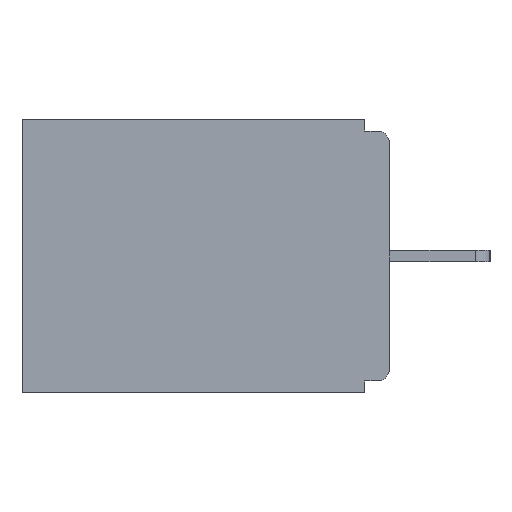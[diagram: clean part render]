
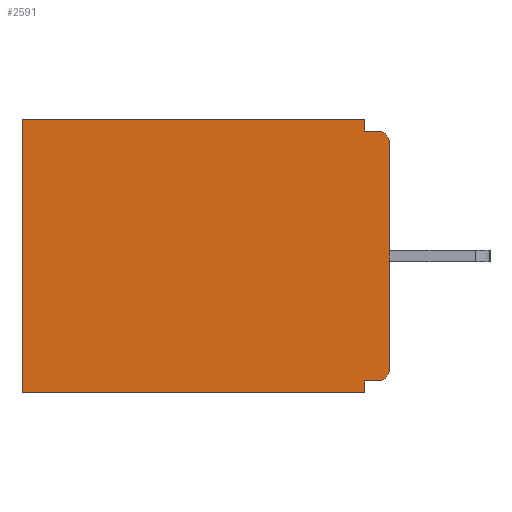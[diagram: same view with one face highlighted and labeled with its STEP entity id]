
A CAD part, left-side view. The second image highlights one B-rep face of the part: STEP entity #2591.
In plain terms, the highlighted planar face has unit normal (-1, 0, 0).
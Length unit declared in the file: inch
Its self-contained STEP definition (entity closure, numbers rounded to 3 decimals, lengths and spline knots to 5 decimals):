
#79 = CARTESIAN_POINT ( 'NONE',  ( 0.298, 0.46, 0. ) ) ;
#199 = DIRECTION ( 'NONE',  ( -1., 0., 0. ) ) ;
#314 = VERTEX_POINT ( 'NONE', #15099 ) ;
#476 = ORIENTED_EDGE ( 'NONE', *, *, #7263, .T. ) ;
#1006 = VERTEX_POINT ( 'NONE', #6099 ) ;
#1531 = EDGE_CURVE ( 'NONE', #8260, #1006, #11961, .T. ) ;
#1885 = DIRECTION ( 'NONE',  ( 0., 0., -1. ) ) ;
#2312 = CARTESIAN_POINT ( 'NONE',  ( 0.298, 0.015, -0.015 ) ) ;
#2591 = ADVANCED_FACE ( 'NONE', ( #6308 ), #11884, .F. ) ;
#3082 = EDGE_CURVE ( 'NONE', #9633, #1006, #24263, .T. ) ;
#3102 = LINE ( 'NONE', #5158, #8505 ) ;
#3244 = AXIS2_PLACEMENT_3D ( 'NONE', #20915, #3994, #19558 ) ;
#3994 = DIRECTION ( 'NONE',  ( 1., 0., 0. ) ) ;
#4077 = ORIENTED_EDGE ( 'NONE', *, *, #24033, .T. ) ;
#4218 = VERTEX_POINT ( 'NONE', #12440 ) ;
#4255 = LINE ( 'NONE', #21909, #19142 ) ;
#4772 = VECTOR ( 'NONE', #18007, 39.37008 ) ;
#4862 = EDGE_CURVE ( 'NONE', #21817, #15502, #5977, .T. ) ;
#5064 = CARTESIAN_POINT ( 'NONE',  ( 0.298, 0., -0.03 ) ) ;
#5158 = CARTESIAN_POINT ( 'NONE',  ( 0.298, 0., 0. ) ) ;
#5640 = ORIENTED_EDGE ( 'NONE', *, *, #14092, .F. ) ;
#5712 = DIRECTION ( 'NONE',  ( 0., 0., -1. ) ) ;
#5977 = LINE ( 'NONE', #21067, #17049 ) ;
#6099 = CARTESIAN_POINT ( 'NONE',  ( 0.298, 0.46, -0.343 ) ) ;
#6211 = CARTESIAN_POINT ( 'NONE',  ( 0.298, 0.031, -0.343 ) ) ;
#6308 = FACE_OUTER_BOUND ( 'NONE', #7611, .T. ) ;
#6361 = AXIS2_PLACEMENT_3D ( 'NONE', #16850, #199, #18939 ) ;
#6556 = CARTESIAN_POINT ( 'NONE',  ( 0.298, 0.031, -0.343 ) ) ;
#7172 = DIRECTION ( 'NONE',  ( -1., 0., 0. ) ) ;
#7263 = EDGE_CURVE ( 'NONE', #314, #9633, #4255, .T. ) ;
#7306 = LINE ( 'NONE', #20403, #14202 ) ;
#7573 = CIRCLE ( 'NONE', #6361, 0.015 ) ;
#7611 = EDGE_LOOP ( 'NONE', ( #19994, #12827, #5640, #476, #18282, #20814, #7846, #9367, #4077, #16255 ) ) ;
#7846 = ORIENTED_EDGE ( 'NONE', *, *, #21912, .F. ) ;
#8206 = CARTESIAN_POINT ( 'NONE',  ( 0.298, 0., -0.328 ) ) ;
#8260 = VERTEX_POINT ( 'NONE', #6211 ) ;
#8505 = VECTOR ( 'NONE', #20128, 39.37008 ) ;
#8909 = CARTESIAN_POINT ( 'NONE',  ( 0.298, 0.015, -0.03 ) ) ;
#9367 = ORIENTED_EDGE ( 'NONE', *, *, #18081, .F. ) ;
#9633 = VERTEX_POINT ( 'NONE', #18733 ) ;
#9982 = EDGE_CURVE ( 'NONE', #17358, #15502, #12496, .T. ) ;
#10052 = DIRECTION ( 'NONE',  ( 0., 1., 0. ) ) ;
#11884 = PLANE ( 'NONE',  #3244 ) ;
#11961 = LINE ( 'NONE', #17741, #4772 ) ;
#12107 = AXIS2_PLACEMENT_3D ( 'NONE', #8909, #7172, #14703 ) ;
#12270 = LINE ( 'NONE', #8206, #17140 ) ;
#12440 = CARTESIAN_POINT ( 'NONE',  ( 0.298, 0.015, -0.328 ) ) ;
#12496 = CIRCLE ( 'NONE', #12107, 0.015 ) ;
#12827 = ORIENTED_EDGE ( 'NONE', *, *, #4862, .F. ) ;
#13541 = VERTEX_POINT ( 'NONE', #20311 ) ;
#14092 = EDGE_CURVE ( 'NONE', #314, #21817, #7306, .T. ) ;
#14202 = VECTOR ( 'NONE', #1885, 39.37008 ) ;
#14595 = DIRECTION ( 'NONE',  ( 0., 1., 0. ) ) ;
#14703 = DIRECTION ( 'NONE',  ( 0., 0., -1. ) ) ;
#14843 = VECTOR ( 'NONE', #17553, 39.37008 ) ;
#15099 = CARTESIAN_POINT ( 'NONE',  ( 0.298, 0.031, 0. ) ) ;
#15502 = VERTEX_POINT ( 'NONE', #2312 ) ;
#15691 = CARTESIAN_POINT ( 'NONE',  ( 0.298, 0.031, -0.328 ) ) ;
#15722 = LINE ( 'NONE', #6556, #14843 ) ;
#16255 = ORIENTED_EDGE ( 'NONE', *, *, #19085, .F. ) ;
#16850 = CARTESIAN_POINT ( 'NONE',  ( 0.298, 0.015, -0.313 ) ) ;
#17049 = VECTOR ( 'NONE', #23396, 39.37008 ) ;
#17140 = VECTOR ( 'NONE', #10052, 39.37008 ) ;
#17358 = VERTEX_POINT ( 'NONE', #5064 ) ;
#17553 = DIRECTION ( 'NONE',  ( 0., 0., -1. ) ) ;
#17741 = CARTESIAN_POINT ( 'NONE',  ( 0.298, 0., -0.343 ) ) ;
#18007 = DIRECTION ( 'NONE',  ( 0., 1., 0. ) ) ;
#18081 = EDGE_CURVE ( 'NONE', #4218, #22318, #12270, .T. ) ;
#18228 = VECTOR ( 'NONE', #5712, 39.37008 ) ;
#18282 = ORIENTED_EDGE ( 'NONE', *, *, #3082, .T. ) ;
#18733 = CARTESIAN_POINT ( 'NONE',  ( 0.298, 0.46, 0. ) ) ;
#18939 = DIRECTION ( 'NONE',  ( 0., 0., -1. ) ) ;
#19085 = EDGE_CURVE ( 'NONE', #17358, #13541, #3102, .T. ) ;
#19142 = VECTOR ( 'NONE', #14595, 39.37008 ) ;
#19558 = DIRECTION ( 'NONE',  ( 0., 0., -1. ) ) ;
#19994 = ORIENTED_EDGE ( 'NONE', *, *, #9982, .T. ) ;
#20128 = DIRECTION ( 'NONE',  ( 0., 0., -1. ) ) ;
#20311 = CARTESIAN_POINT ( 'NONE',  ( 0.298, 0., -0.313 ) ) ;
#20403 = CARTESIAN_POINT ( 'NONE',  ( 0.298, 0.031, -0.343 ) ) ;
#20673 = CARTESIAN_POINT ( 'NONE',  ( 0.298, 0.031, -0.015 ) ) ;
#20814 = ORIENTED_EDGE ( 'NONE', *, *, #1531, .F. ) ;
#20915 = CARTESIAN_POINT ( 'NONE',  ( 0.298, 0., 0. ) ) ;
#21067 = CARTESIAN_POINT ( 'NONE',  ( 0.298, 0., -0.015 ) ) ;
#21817 = VERTEX_POINT ( 'NONE', #20673 ) ;
#21909 = CARTESIAN_POINT ( 'NONE',  ( 0.298, 0., 0. ) ) ;
#21912 = EDGE_CURVE ( 'NONE', #22318, #8260, #15722, .T. ) ;
#22318 = VERTEX_POINT ( 'NONE', #15691 ) ;
#23396 = DIRECTION ( 'NONE',  ( 0., -1., 0. ) ) ;
#24033 = EDGE_CURVE ( 'NONE', #4218, #13541, #7573, .T. ) ;
#24263 = LINE ( 'NONE', #79, #18228 ) ;
